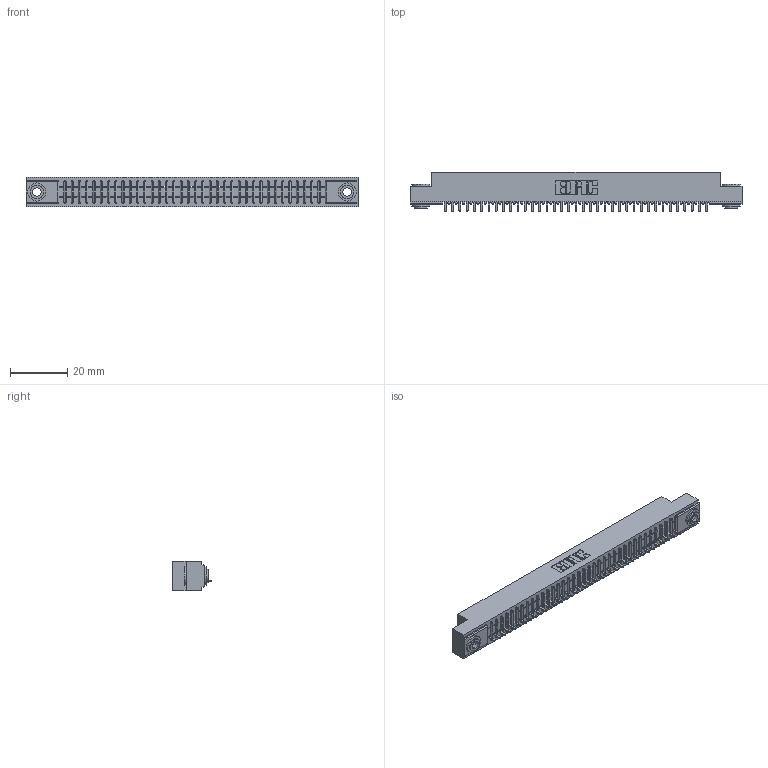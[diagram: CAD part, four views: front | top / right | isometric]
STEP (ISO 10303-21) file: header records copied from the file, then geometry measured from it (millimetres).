
FILE_DESCRIPTION (( 'STEP AP203' ), '1' );
FILE_NAME ('341-037-524-103.STEP', '2018-08-06T23:06:48', ( '' ), ( '' ), 'SwSTEP 2.0', 'SolidWorks 2016', '' );
FILE_SCHEMA (( 'CONFIG_CONTROL_DESIGN' ));
Length unit declared in the file: inch
Products named in the file (4): 341-037-524-103; 341 Part_.156 (3.96) Dia Mounting Holes; 341-292-001_341-292-124; 345-250-002_345-250-002-102
Assembly tree (40 placements, depth 2):
  341-037-524-103
    341 Part_.156 (3.96) Dia Mounting Holes
    341-292-001_341-292-124  x37
    345-250-002_345-250-002-102  x2
Bounding box: 116.2 x 13.64 x 10.16 mm (x, y, z)
Volume: 8309.8 mm3; surface area: 12923.6 mm2
Topology: 40 solids, 40 shells, 3202 faces, 9197 edges, 5902 vertices
Faces by surface type: plane 1979, cylinder 1067, sphere 76, torus 72, cone 8
Entity records: 45325 total; most frequent: CARTESIAN_POINT 7675, ORIENTED_EDGE 7654, DIRECTION 7429, EDGE_CURVE 3827, LINE 3077, VECTOR 3077, VERTEX_POINT 2422, AXIS2_PLACEMENT_3D 2176
